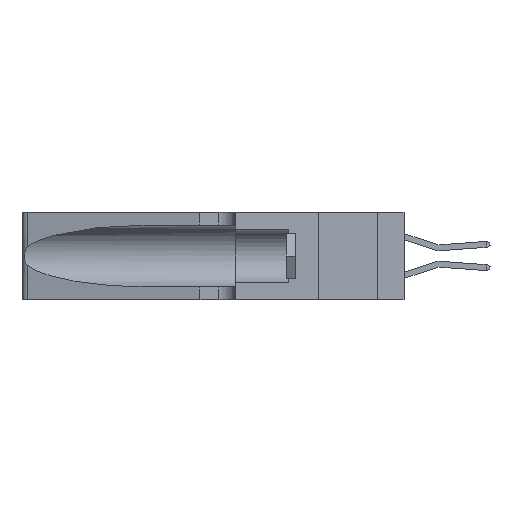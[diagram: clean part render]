
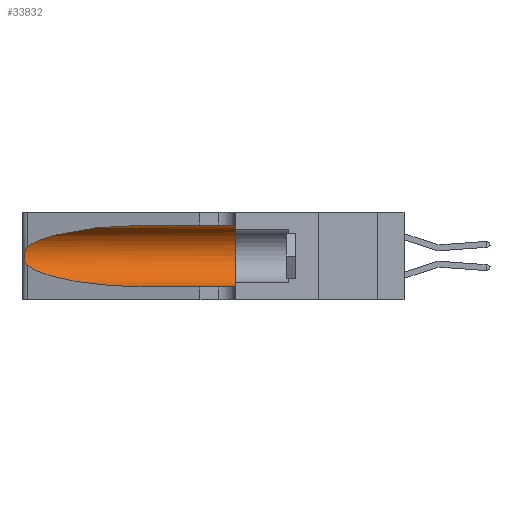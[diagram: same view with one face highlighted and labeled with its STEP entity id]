
A CAD part, left-side view. The second image highlights one B-rep face of the part: STEP entity #33832.
In plain terms, the highlighted cylindrical face has radius 3.308 mm (diameter 6.617 mm), a partial arc.
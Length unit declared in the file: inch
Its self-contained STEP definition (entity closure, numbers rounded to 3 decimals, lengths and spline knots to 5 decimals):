
#336 = ORIENTED_EDGE ( 'NONE', *, *, #19910, .T. ) ;
#783 = CARTESIAN_POINT ( 'NONE',  ( 0.25789, 1.23486, 0.15765 ) ) ;
#1936 = CARTESIAN_POINT ( 'NONE',  ( 0.1305, 0.72297, 0.31525 ) ) ;
#2111 = ORIENTED_EDGE ( 'NONE', *, *, #15509, .T. ) ;
#3251 = ORIENTED_EDGE ( 'NONE', *, *, #27076, .F. ) ;
#3383 = CARTESIAN_POINT ( 'NONE',  ( 0.25487, 1.22718, 0.22369 ) ) ;
#3430 = DIRECTION ( 'NONE',  ( 0., -1., 0. ) ) ;
#3497 = CARTESIAN_POINT ( 'NONE',  ( 0.25555, 1.22993, 0.14849 ) ) ;
#4012 = VERTEX_POINT ( 'NONE', #14851 ) ;
#4559 = AXIS2_PLACEMENT_3D ( 'NONE', #16708, #3430, #6181 ) ;
#4691 = FACE_OUTER_BOUND ( 'NONE', #23538, .T. ) ;
#6181 = DIRECTION ( 'NONE',  ( 0., 0., -1. ) ) ;
#7976 = VERTEX_POINT ( 'NONE', #25773 ) ;
#8284 = B_SPLINE_CURVE_WITH_KNOTS ( 'NONE', 3,
 ( #3383, #19360, #24529, #8885, #27098, #11584, #29699, #14263, #32283, #16890, #783, #19472, #3497, #22058 ),
 .UNSPECIFIED., .F., .F.,
 ( 4, 2, 2, 2, 2, 2, 4 ),
 ( 0., 0.00027, 0.00053, 0.00107, 0.0016, 0.00187, 0.00214 ),
 .UNSPECIFIED. ) ;
#8885 = CARTESIAN_POINT ( 'NONE',  ( 0.25787, 1.23484, 0.2124 ) ) ;
#10344 = CARTESIAN_POINT ( 'NONE',  ( 0.2373, 1.15595, 0.28018 ) ) ;
#11184 = EDGE_CURVE ( 'NONE', #7976, #29447, #20209, .T. ) ;
#11584 = CARTESIAN_POINT ( 'NONE',  ( 0.26018, 1.23835, 0.19895 ) ) ;
#11634 = CARTESIAN_POINT ( 'NONE',  ( 0.1305, 0.72297, 0.05475 ) ) ;
#11701 = AXIS2_PLACEMENT_3D ( 'NONE', #15973, #33940, #18556 ) ;
#11940 =( BOUNDED_CURVE ( )  B_SPLINE_CURVE ( 3, ( #24574, #29627, #27144, #11634 ),
 .UNSPECIFIED., .F., .F. ) 
 B_SPLINE_CURVE_WITH_KNOTS ( ( 4, 4 ),
 ( 3.44316, 4.71239 ),
 .UNSPECIFIED. ) 
 CURVE ( )  GEOMETRIC_REPRESENTATION_ITEM ( )  RATIONAL_B_SPLINE_CURVE ( ( 1., 0.87, 0.87, 1. ) ) 
 REPRESENTATION_ITEM ( '' )  );
#13008 = CARTESIAN_POINT ( 'NONE',  ( 0.1305, 0.72297, 0.31525 ) ) ;
#13135 = CIRCLE ( 'NONE', #11701, 0.13025 ) ;
#14137 = ORIENTED_EDGE ( 'NONE', *, *, #11184, .T. ) ;
#14182 = EDGE_CURVE ( 'NONE', #16763, #29447, #13135, .T. ) ;
#14263 = CARTESIAN_POINT ( 'NONE',  ( 0.26075, 1.23896, 0.178 ) ) ;
#14423 = ORIENTED_EDGE ( 'NONE', *, *, #29677, .T. ) ;
#14511 =( BOUNDED_CURVE ( )  B_SPLINE_CURVE ( 3, ( #13008, #15563, #10344, #31081 ),
 .UNSPECIFIED., .F., .F. ) 
 B_SPLINE_CURVE_WITH_KNOTS ( ( 4, 4 ),
 ( 1.5708, 2.84003 ),
 .UNSPECIFIED. ) 
 CURVE ( )  GEOMETRIC_REPRESENTATION_ITEM ( )  RATIONAL_B_SPLINE_CURVE ( ( 1., 0.87, 0.87, 1. ) ) 
 REPRESENTATION_ITEM ( '' )  );
#14851 = CARTESIAN_POINT ( 'NONE',  ( 0.25487, 1.22718, 0.14631 ) ) ;
#15509 = EDGE_CURVE ( 'NONE', #23252, #24316, #14511, .T. ) ;
#15563 = CARTESIAN_POINT ( 'NONE',  ( 0.18966, 0.96281, 0.31525 ) ) ;
#15583 = CARTESIAN_POINT ( 'NONE',  ( 0.1305, 1.61858, 0.31525 ) ) ;
#15973 = CARTESIAN_POINT ( 'NONE',  ( 0.1305, 0.35, 0.185 ) ) ;
#16708 = CARTESIAN_POINT ( 'NONE',  ( 0.1305, 1.61858, 0.185 ) ) ;
#16763 = VERTEX_POINT ( 'NONE', #28540 ) ;
#16890 = CARTESIAN_POINT ( 'NONE',  ( 0.25856, 1.23593, 0.16098 ) ) ;
#18556 = DIRECTION ( 'NONE',  ( 0., 0., 1. ) ) ;
#19360 = CARTESIAN_POINT ( 'NONE',  ( 0.25555, 1.22994, 0.2215 ) ) ;
#19472 = CARTESIAN_POINT ( 'NONE',  ( 0.25639, 1.23186, 0.15144 ) ) ;
#19910 = EDGE_CURVE ( 'NONE', #24316, #4012, #8284, .T. ) ;
#20209 = LINE ( 'NONE', #30751, #33071 ) ;
#20381 = LINE ( 'NONE', #15583, #34027 ) ;
#22058 = CARTESIAN_POINT ( 'NONE',  ( 0.25487, 1.22718, 0.14631 ) ) ;
#23252 = VERTEX_POINT ( 'NONE', #1936 ) ;
#23538 = EDGE_LOOP ( 'NONE', ( #2111, #336, #14423, #14137, #31429, #3251 ) ) ;
#24316 = VERTEX_POINT ( 'NONE', #30042 ) ;
#24529 = CARTESIAN_POINT ( 'NONE',  ( 0.25639, 1.23184, 0.21858 ) ) ;
#24574 = CARTESIAN_POINT ( 'NONE',  ( 0.25487, 1.22718, 0.14631 ) ) ;
#25773 = CARTESIAN_POINT ( 'NONE',  ( 0.1305, 0.72297, 0.05475 ) ) ;
#27076 = EDGE_CURVE ( 'NONE', #23252, #16763, #20381, .T. ) ;
#27098 = CARTESIAN_POINT ( 'NONE',  ( 0.25854, 1.2359, 0.20912 ) ) ;
#27144 = CARTESIAN_POINT ( 'NONE',  ( 0.18966, 0.96281, 0.05475 ) ) ;
#28540 = CARTESIAN_POINT ( 'NONE',  ( 0.1305, 0.35, 0.31525 ) ) ;
#28731 = CARTESIAN_POINT ( 'NONE',  ( 0.1305, 0.35, 0.05475 ) ) ;
#29299 = CYLINDRICAL_SURFACE ( 'NONE', #4559, 0.13025 ) ;
#29447 = VERTEX_POINT ( 'NONE', #28731 ) ;
#29627 = CARTESIAN_POINT ( 'NONE',  ( 0.2373, 1.15595, 0.08982 ) ) ;
#29677 = EDGE_CURVE ( 'NONE', #4012, #7976, #11940, .T. ) ;
#29699 = CARTESIAN_POINT ( 'NONE',  ( 0.26075, 1.23896, 0.19203 ) ) ;
#30042 = CARTESIAN_POINT ( 'NONE',  ( 0.25487, 1.22718, 0.22369 ) ) ;
#30751 = CARTESIAN_POINT ( 'NONE',  ( 0.1305, 1.61858, 0.05475 ) ) ;
#31081 = CARTESIAN_POINT ( 'NONE',  ( 0.25487, 1.22718, 0.22369 ) ) ;
#31429 = ORIENTED_EDGE ( 'NONE', *, *, #14182, .F. ) ;
#32283 = CARTESIAN_POINT ( 'NONE',  ( 0.26017, 1.23833, 0.17102 ) ) ;
#33071 = VECTOR ( 'NONE', #33345, 39.37008 ) ;
#33345 = DIRECTION ( 'NONE',  ( 0., -1., 0. ) ) ;
#33563 = DIRECTION ( 'NONE',  ( 0., -1., 0. ) ) ;
#33832 = ADVANCED_FACE ( 'NONE', ( #4691 ), #29299, .F. ) ;
#33940 = DIRECTION ( 'NONE',  ( 0., 1., 0. ) ) ;
#34027 = VECTOR ( 'NONE', #33563, 39.37008 ) ;
